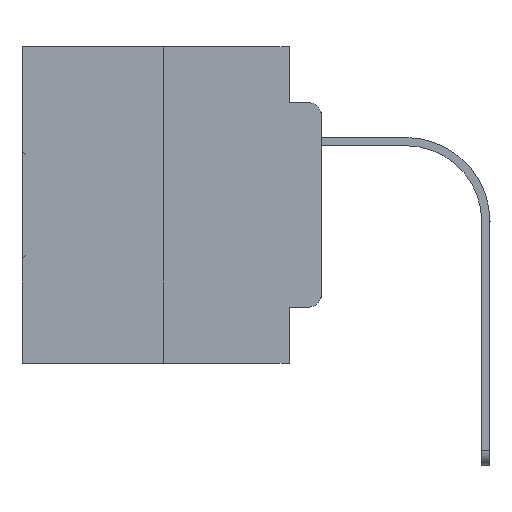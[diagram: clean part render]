
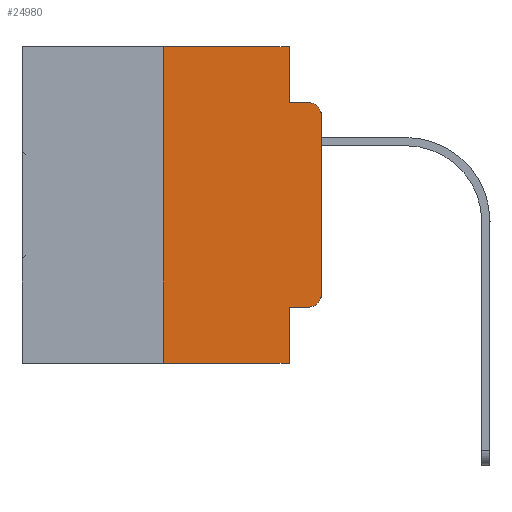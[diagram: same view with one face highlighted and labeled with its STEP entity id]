
A CAD part, left-side view. The second image highlights one B-rep face of the part: STEP entity #24980.
In plain terms, the highlighted planar face has unit normal (-1, 0, 0).
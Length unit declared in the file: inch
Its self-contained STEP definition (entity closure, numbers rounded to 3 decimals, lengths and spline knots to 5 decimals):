
#53 = EDGE_CURVE ( 'NONE', #2449, #21005, #10292, .T. ) ;
#1974 = CARTESIAN_POINT ( 'NONE',  ( 0., 0.051, 0. ) ) ;
#2416 = DIRECTION ( 'NONE',  ( 0., 0., 1. ) ) ;
#2449 = VERTEX_POINT ( 'NONE', #23033 ) ;
#2466 = LINE ( 'NONE', #14418, #7330 ) ;
#2587 = CARTESIAN_POINT ( 'NONE',  ( 0., 0.02, -0.1085 ) ) ;
#3033 = EDGE_CURVE ( 'NONE', #22245, #24573, #6833, .T. ) ;
#3370 = CARTESIAN_POINT ( 'NONE',  ( 0., 0.02, -0.3915 ) ) ;
#3382 = DIRECTION ( 'NONE',  ( 1., 0., 0. ) ) ;
#3386 = VERTEX_POINT ( 'NONE', #14103 ) ;
#3701 = PLANE ( 'NONE',  #6628 ) ;
#3982 = LINE ( 'NONE', #29730, #6976 ) ;
#4892 = CARTESIAN_POINT ( 'NONE',  ( 0., 0., -0.1085 ) ) ;
#5068 = AXIS2_PLACEMENT_3D ( 'NONE', #2587, #19041, #23236 ) ;
#5688 = CARTESIAN_POINT ( 'NONE',  ( 0., 0.02, -0.0885 ) ) ;
#5709 = CARTESIAN_POINT ( 'NONE',  ( 0., 0.473, 0. ) ) ;
#5828 = CARTESIAN_POINT ( 'NONE',  ( 0., 0.25, 0. ) ) ;
#6099 = CARTESIAN_POINT ( 'NONE',  ( 0., 0., -0.3915 ) ) ;
#6628 = AXIS2_PLACEMENT_3D ( 'NONE', #5709, #3382, #17491 ) ;
#6833 = LINE ( 'NONE', #14140, #30058 ) ;
#6976 = VECTOR ( 'NONE', #28020, 39.37008 ) ;
#7140 = DIRECTION ( 'NONE',  ( 0., -1., 0. ) ) ;
#7227 = LINE ( 'NONE', #14231, #30624 ) ;
#7330 = VECTOR ( 'NONE', #23262, 39.37008 ) ;
#7432 = ORIENTED_EDGE ( 'NONE', *, *, #18204, .F. ) ;
#7951 = CARTESIAN_POINT ( 'NONE',  ( 0., 0.25, 0. ) ) ;
#8275 = VECTOR ( 'NONE', #15292, 39.37008 ) ;
#8484 = ORIENTED_EDGE ( 'NONE', *, *, #18753, .T. ) ;
#9012 = ORIENTED_EDGE ( 'NONE', *, *, #22719, .F. ) ;
#9103 = DIRECTION ( 'NONE',  ( 0., 0., -1. ) ) ;
#9279 = ORIENTED_EDGE ( 'NONE', *, *, #25449, .F. ) ;
#10143 = DIRECTION ( 'NONE',  ( 0., -1., 0. ) ) ;
#10196 = VERTEX_POINT ( 'NONE', #27892 ) ;
#10292 = LINE ( 'NONE', #16658, #25107 ) ;
#10593 = CARTESIAN_POINT ( 'NONE',  ( 0., 0.051, -0.5 ) ) ;
#10666 = FACE_OUTER_BOUND ( 'NONE', #16266, .T. ) ;
#10931 = VERTEX_POINT ( 'NONE', #5688 ) ;
#11088 = EDGE_CURVE ( 'NONE', #13349, #3386, #3982, .T. ) ;
#11524 = ORIENTED_EDGE ( 'NONE', *, *, #3033, .F. ) ;
#11766 = VECTOR ( 'NONE', #9103, 39.37008 ) ;
#11795 = CARTESIAN_POINT ( 'NONE',  ( 0., 0.051, -0.4115 ) ) ;
#13349 = VERTEX_POINT ( 'NONE', #11795 ) ;
#13722 = EDGE_CURVE ( 'NONE', #30309, #10931, #29844, .T. ) ;
#14103 = CARTESIAN_POINT ( 'NONE',  ( 0., 0.02, -0.4115 ) ) ;
#14140 = CARTESIAN_POINT ( 'NONE',  ( 0., 0.473, 0. ) ) ;
#14231 = CARTESIAN_POINT ( 'NONE',  ( 0., 0.051, 0. ) ) ;
#14418 = CARTESIAN_POINT ( 'NONE',  ( 0., 0.051, -0.0885 ) ) ;
#15292 = DIRECTION ( 'NONE',  ( 0., 0., 1. ) ) ;
#15806 = AXIS2_PLACEMENT_3D ( 'NONE', #3370, #26795, #17634 ) ;
#16266 = EDGE_LOOP ( 'NONE', ( #21093, #23933, #7432, #9279, #11524, #9012, #21293, #20894, #25116, #8484 ) ) ;
#16658 = CARTESIAN_POINT ( 'NONE',  ( 0., 0.473, -0.5 ) ) ;
#17068 = CARTESIAN_POINT ( 'NONE',  ( 0., 0.051, 0. ) ) ;
#17345 = EDGE_CURVE ( 'NONE', #13349, #21005, #25560, .T. ) ;
#17491 = DIRECTION ( 'NONE',  ( 0., 0., -1. ) ) ;
#17634 = DIRECTION ( 'NONE',  ( 0., 0., -1. ) ) ;
#18204 = EDGE_CURVE ( 'NONE', #10196, #10931, #2466, .T. ) ;
#18753 = EDGE_CURVE ( 'NONE', #3386, #23134, #29673, .T. ) ;
#19017 = LINE ( 'NONE', #28494, #23789 ) ;
#19041 = DIRECTION ( 'NONE',  ( -1., 0., 0. ) ) ;
#20369 = EDGE_CURVE ( 'NONE', #23134, #30309, #19017, .T. ) ;
#20894 = ORIENTED_EDGE ( 'NONE', *, *, #17345, .F. ) ;
#21005 = VERTEX_POINT ( 'NONE', #10593 ) ;
#21093 = ORIENTED_EDGE ( 'NONE', *, *, #20369, .T. ) ;
#21293 = ORIENTED_EDGE ( 'NONE', *, *, #53, .T. ) ;
#22245 = VERTEX_POINT ( 'NONE', #7951 ) ;
#22719 = EDGE_CURVE ( 'NONE', #2449, #22245, #27248, .T. ) ;
#23033 = CARTESIAN_POINT ( 'NONE',  ( 0., 0.25, -0.5 ) ) ;
#23134 = VERTEX_POINT ( 'NONE', #6099 ) ;
#23236 = DIRECTION ( 'NONE',  ( 0., 0., -1. ) ) ;
#23262 = DIRECTION ( 'NONE',  ( 0., -1., 0. ) ) ;
#23789 = VECTOR ( 'NONE', #2416, 39.37008 ) ;
#23933 = ORIENTED_EDGE ( 'NONE', *, *, #13722, .T. ) ;
#24573 = VERTEX_POINT ( 'NONE', #17068 ) ;
#24980 = ADVANCED_FACE ( 'NONE', ( #10666 ), #3701, .F. ) ;
#25107 = VECTOR ( 'NONE', #10143, 39.37008 ) ;
#25116 = ORIENTED_EDGE ( 'NONE', *, *, #11088, .T. ) ;
#25449 = EDGE_CURVE ( 'NONE', #24573, #10196, #7227, .T. ) ;
#25560 = LINE ( 'NONE', #1974, #11766 ) ;
#26795 = DIRECTION ( 'NONE',  ( -1., 0., 0. ) ) ;
#27248 = LINE ( 'NONE', #5828, #8275 ) ;
#27892 = CARTESIAN_POINT ( 'NONE',  ( 0., 0.051, -0.0885 ) ) ;
#28020 = DIRECTION ( 'NONE',  ( 0., -1., 0. ) ) ;
#28494 = CARTESIAN_POINT ( 'NONE',  ( 0., 0., 0. ) ) ;
#28659 = DIRECTION ( 'NONE',  ( 0., 0., -1. ) ) ;
#29673 = CIRCLE ( 'NONE', #15806, 0.02 ) ;
#29730 = CARTESIAN_POINT ( 'NONE',  ( 0., 0.051, -0.4115 ) ) ;
#29844 = CIRCLE ( 'NONE', #5068, 0.02 ) ;
#30058 = VECTOR ( 'NONE', #7140, 39.37008 ) ;
#30309 = VERTEX_POINT ( 'NONE', #4892 ) ;
#30624 = VECTOR ( 'NONE', #28659, 39.37008 ) ;
